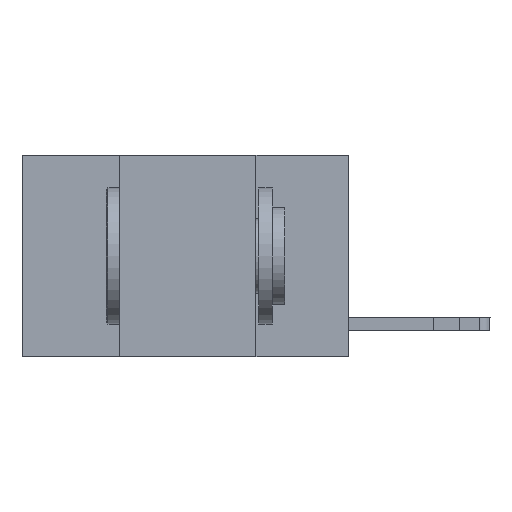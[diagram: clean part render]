
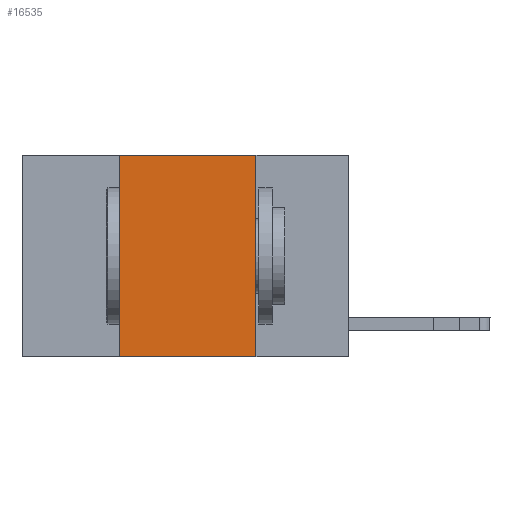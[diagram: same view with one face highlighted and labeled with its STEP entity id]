
A CAD part, left-side view. The second image highlights one B-rep face of the part: STEP entity #16535.
In plain terms, the highlighted planar face has unit normal (-1, 0, 0).
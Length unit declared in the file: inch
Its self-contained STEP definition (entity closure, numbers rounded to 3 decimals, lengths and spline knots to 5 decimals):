
#542 = CARTESIAN_POINT ( 'NONE',  ( 0., 0.6, 0. ) ) ;
#676 = FACE_OUTER_BOUND ( 'NONE', #4231, .T. ) ;
#875 = ORIENTED_EDGE ( 'NONE', *, *, #8594, .T. ) ;
#2275 = VERTEX_POINT ( 'NONE', #21181 ) ;
#2981 = VECTOR ( 'NONE', #23302, 39.37008 ) ;
#4231 = EDGE_LOOP ( 'NONE', ( #24351, #16529, #14206, #875 ) ) ;
#4473 = DIRECTION ( 'NONE',  ( 0., -1., 0. ) ) ;
#5488 = CARTESIAN_POINT ( 'NONE',  ( 0., 0.17, 0. ) ) ;
#6247 = EDGE_CURVE ( 'NONE', #2275, #24925, #24027, .T. ) ;
#6699 = EDGE_CURVE ( 'NONE', #16876, #2275, #23012, .T. ) ;
#7949 = CARTESIAN_POINT ( 'NONE',  ( 0., 0.42, -0.37 ) ) ;
#8594 = EDGE_CURVE ( 'NONE', #19682, #24925, #8673, .T. ) ;
#8673 = LINE ( 'NONE', #15025, #2981 ) ;
#8904 = PLANE ( 'NONE',  #12644 ) ;
#9719 = DIRECTION ( 'NONE',  ( 0., 0., 1. ) ) ;
#10571 = VECTOR ( 'NONE', #9719, 39.37008 ) ;
#12644 = AXIS2_PLACEMENT_3D ( 'NONE', #542, #17145, #14455 ) ;
#14206 = ORIENTED_EDGE ( 'NONE', *, *, #19573, .F. ) ;
#14455 = DIRECTION ( 'NONE',  ( 0., 0., -1. ) ) ;
#15025 = CARTESIAN_POINT ( 'NONE',  ( 0., 0.6, -0.37 ) ) ;
#16529 = ORIENTED_EDGE ( 'NONE', *, *, #6699, .F. ) ;
#16535 = ADVANCED_FACE ( 'NONE', ( #676 ), #8904, .F. ) ;
#16876 = VERTEX_POINT ( 'NONE', #19404 ) ;
#17145 = DIRECTION ( 'NONE',  ( 1., 0., 0. ) ) ;
#17993 = VECTOR ( 'NONE', #24167, 39.37008 ) ;
#19404 = CARTESIAN_POINT ( 'NONE',  ( 0., 0.42, 0. ) ) ;
#19573 = EDGE_CURVE ( 'NONE', #19682, #16876, #23920, .T. ) ;
#19682 = VERTEX_POINT ( 'NONE', #7949 ) ;
#19884 = CARTESIAN_POINT ( 'NONE',  ( 0., 0.17, -0.37 ) ) ;
#19988 = CARTESIAN_POINT ( 'NONE',  ( 0., 0.42, 0. ) ) ;
#20086 = CARTESIAN_POINT ( 'NONE',  ( 0., 0.6, 0. ) ) ;
#21181 = CARTESIAN_POINT ( 'NONE',  ( 0., 0.17, 0. ) ) ;
#23012 = LINE ( 'NONE', #20086, #23647 ) ;
#23302 = DIRECTION ( 'NONE',  ( 0., -1., 0. ) ) ;
#23647 = VECTOR ( 'NONE', #4473, 39.37008 ) ;
#23920 = LINE ( 'NONE', #19988, #10571 ) ;
#24027 = LINE ( 'NONE', #5488, #17993 ) ;
#24167 = DIRECTION ( 'NONE',  ( 0., 0., -1. ) ) ;
#24351 = ORIENTED_EDGE ( 'NONE', *, *, #6247, .F. ) ;
#24925 = VERTEX_POINT ( 'NONE', #19884 ) ;
